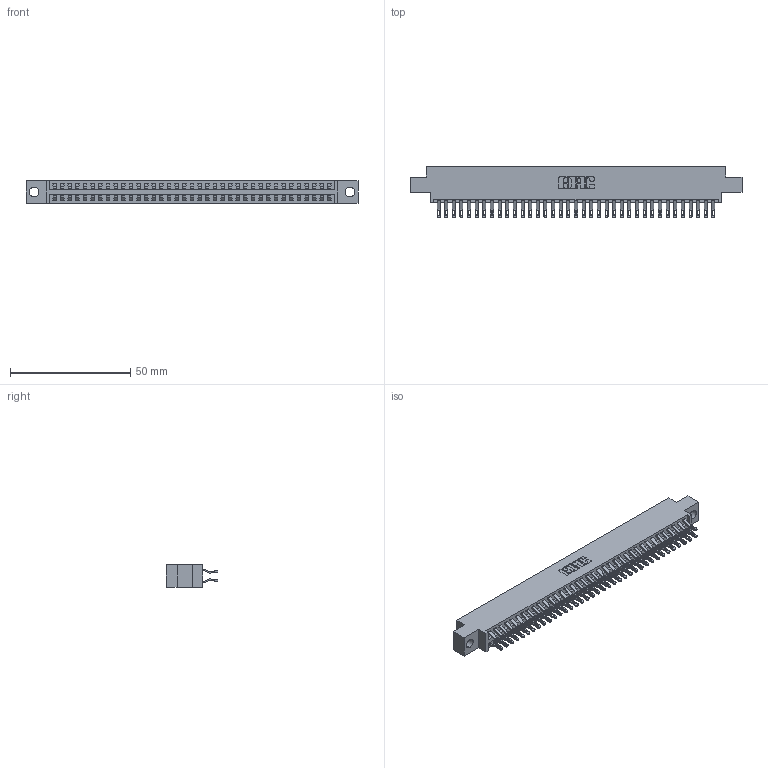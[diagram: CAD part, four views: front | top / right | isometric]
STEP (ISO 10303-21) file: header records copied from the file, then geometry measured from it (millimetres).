
FILE_DESCRIPTION (( 'STEP AP203' ), '1' );
FILE_NAME ('346-074-555-804.STEP', '2022-05-25T03:04:01', ( '' ), ( '' ), 'SwSTEP 2.0', 'SolidWorks 2020', '' );
FILE_SCHEMA (( 'CONFIG_CONTROL_DESIGN' ));
Length unit declared in the file: inch
Products named in the file (3): 346-074-555-804; 345-292-001_555 Tail; 346 Part_0.170 Offset - 0.156 Dia-TH
Assembly tree (75 placements, depth 2):
  346-074-555-804
    346 Part_0.170 Offset - 0.156 Dia-TH
    345-292-001_555 Tail  x74
Bounding box: 138.05 x 21.46 x 9.4 mm (x, y, z)
Volume: 13376.7 mm3; surface area: 19101.3 mm2
Topology: 75 solids, 75 shells, 4432 faces, 13919 edges, 9278 vertices
Faces by surface type: plane 2536, cylinder 1896
Entity records: 25697 total; most frequent: CARTESIAN_POINT 4284, ORIENTED_EDGE 4186, DIRECTION 3793, EDGE_CURVE 2093, VECTOR 1793, LINE 1793, VERTEX_POINT 1394, AXIS2_PLACEMENT_3D 1000
